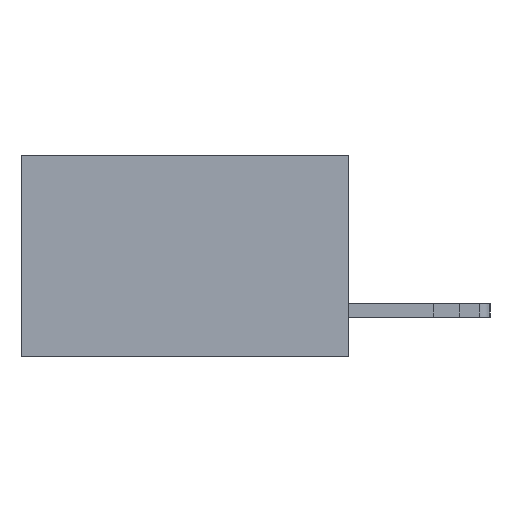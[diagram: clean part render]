
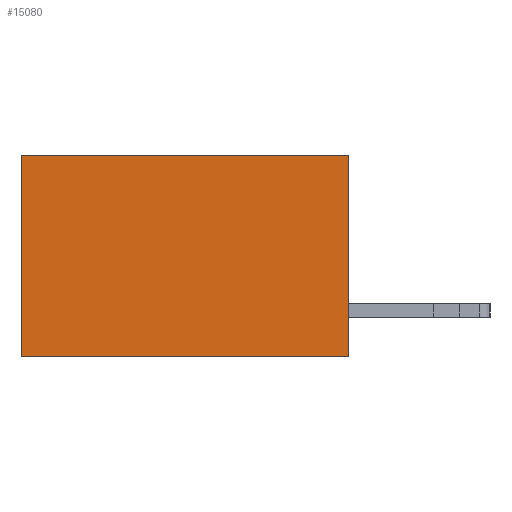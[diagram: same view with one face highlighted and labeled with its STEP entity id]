
A CAD part, left-side view. The second image highlights one B-rep face of the part: STEP entity #15080.
In plain terms, the highlighted planar face has unit normal (-1, 0, 0).
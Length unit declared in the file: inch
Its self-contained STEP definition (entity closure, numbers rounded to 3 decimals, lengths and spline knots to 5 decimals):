
#194 = CARTESIAN_POINT ( 'NONE',  ( 0.2615, 0., 0. ) ) ;
#205 = PLANE ( 'NONE',  #14979 ) ;
#365 = VECTOR ( 'NONE', #6468, 39.37008 ) ;
#423 = FACE_OUTER_BOUND ( 'NONE', #8924, .T. ) ;
#530 = VECTOR ( 'NONE', #9116, 39.37008 ) ;
#1263 = LINE ( 'NONE', #10269, #11110 ) ;
#1336 = EDGE_CURVE ( 'NONE', #8360, #7096, #4788, .T. ) ;
#1620 = DIRECTION ( 'NONE',  ( 0., 0., -1. ) ) ;
#2411 = LINE ( 'NONE', #16368, #12998 ) ;
#3277 = ORIENTED_EDGE ( 'NONE', *, *, #5836, .T. ) ;
#3912 = VERTEX_POINT ( 'NONE', #9409 ) ;
#4788 = LINE ( 'NONE', #9341, #530 ) ;
#5597 = DIRECTION ( 'NONE',  ( 0., 0., -1. ) ) ;
#5836 = EDGE_CURVE ( 'NONE', #3912, #7096, #1263, .T. ) ;
#6468 = DIRECTION ( 'NONE',  ( 0., 1., 0. ) ) ;
#7096 = VERTEX_POINT ( 'NONE', #16338 ) ;
#7309 = CARTESIAN_POINT ( 'NONE',  ( 0.2615, 0., -0.37 ) ) ;
#8360 = VERTEX_POINT ( 'NONE', #7309 ) ;
#8661 = ORIENTED_EDGE ( 'NONE', *, *, #15568, .F. ) ;
#8698 = CARTESIAN_POINT ( 'NONE',  ( 0.2615, 0., -0.37 ) ) ;
#8924 = EDGE_LOOP ( 'NONE', ( #3277, #9936, #8661, #9965 ) ) ;
#9116 = DIRECTION ( 'NONE',  ( 0., 1., 0. ) ) ;
#9341 = CARTESIAN_POINT ( 'NONE',  ( 0.2615, 0., -0.37 ) ) ;
#9409 = CARTESIAN_POINT ( 'NONE',  ( 0.2615, 0.6, 0. ) ) ;
#9629 = VERTEX_POINT ( 'NONE', #194 ) ;
#9936 = ORIENTED_EDGE ( 'NONE', *, *, #1336, .F. ) ;
#9965 = ORIENTED_EDGE ( 'NONE', *, *, #10607, .T. ) ;
#10076 = DIRECTION ( 'NONE',  ( 1., 0., 0. ) ) ;
#10119 = DIRECTION ( 'NONE',  ( 0., 0., -1. ) ) ;
#10269 = CARTESIAN_POINT ( 'NONE',  ( 0.2615, 0.6, -0.37 ) ) ;
#10607 = EDGE_CURVE ( 'NONE', #9629, #3912, #15055, .T. ) ;
#11110 = VECTOR ( 'NONE', #10119, 39.37008 ) ;
#12998 = VECTOR ( 'NONE', #5597, 39.37008 ) ;
#14610 = CARTESIAN_POINT ( 'NONE',  ( 0.2615, 0., 0. ) ) ;
#14979 = AXIS2_PLACEMENT_3D ( 'NONE', #8698, #10076, #1620 ) ;
#15055 = LINE ( 'NONE', #14610, #365 ) ;
#15080 = ADVANCED_FACE ( 'NONE', ( #423 ), #205, .F. ) ;
#15568 = EDGE_CURVE ( 'NONE', #9629, #8360, #2411, .T. ) ;
#16338 = CARTESIAN_POINT ( 'NONE',  ( 0.2615, 0.6, -0.37 ) ) ;
#16368 = CARTESIAN_POINT ( 'NONE',  ( 0.2615, 0., -0.37 ) ) ;
